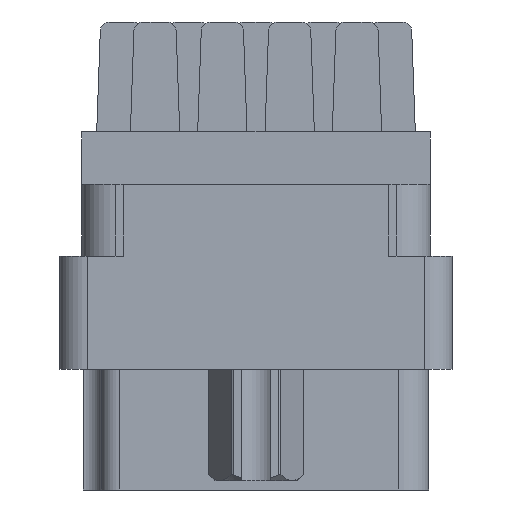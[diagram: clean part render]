
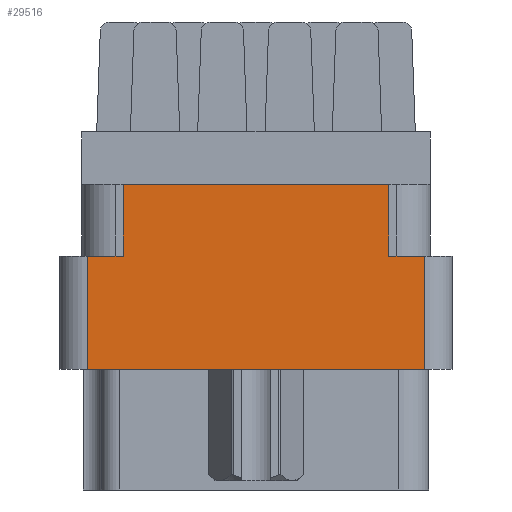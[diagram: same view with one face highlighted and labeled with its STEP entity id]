
A CAD part, left-side view. The second image highlights one B-rep face of the part: STEP entity #29516.
In plain terms, the highlighted planar face has unit normal (-1, 0, 0).
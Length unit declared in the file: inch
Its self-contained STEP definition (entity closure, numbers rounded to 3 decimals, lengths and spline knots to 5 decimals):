
#1002 = LINE ( 'NONE', #26034, #19584 ) ;
#2303 = CARTESIAN_POINT ( 'NONE',  ( -1., 0.376, -0.529 ) ) ;
#3102 = VECTOR ( 'NONE', #3539, 39.37008 ) ;
#3539 = DIRECTION ( 'NONE',  ( 0., -1., 0. ) ) ;
#3864 = CARTESIAN_POINT ( 'NONE',  ( -1., -0.376, -0.277 ) ) ;
#3985 = VECTOR ( 'NONE', #44143, 39.37008 ) ;
#4215 = CARTESIAN_POINT ( 'NONE',  ( -1., -0.438, -0.798 ) ) ;
#5574 = CARTESIAN_POINT ( 'NONE',  ( -1., -0.376, -0.529 ) ) ;
#5891 = VERTEX_POINT ( 'NONE', #5574 ) ;
#5908 = EDGE_CURVE ( 'NONE', #46362, #29553, #9421, .T. ) ;
#5971 = EDGE_CURVE ( 'NONE', #5891, #8321, #36577, .T. ) ;
#6487 = DIRECTION ( 'NONE',  ( 0., 0., -1. ) ) ;
#8308 = FACE_OUTER_BOUND ( 'NONE', #11083, .T. ) ;
#8321 = VERTEX_POINT ( 'NONE', #3864 ) ;
#9182 = CARTESIAN_POINT ( 'NONE',  ( -1., 0., -0.277 ) ) ;
#9421 = LINE ( 'NONE', #9182, #23966 ) ;
#9979 = ORIENTED_EDGE ( 'NONE', *, *, #21699, .F. ) ;
#11083 = EDGE_LOOP ( 'NONE', ( #22367, #42477, #26662, #16470, #28057, #23866, #9979, #14936 ) ) ;
#11517 = EDGE_CURVE ( 'NONE', #46362, #23050, #45489, .T. ) ;
#11698 = CARTESIAN_POINT ( 'NONE',  ( -1., 0.296, -0.277 ) ) ;
#13220 = VECTOR ( 'NONE', #36342, 39.37008 ) ;
#14936 = ORIENTED_EDGE ( 'NONE', *, *, #29615, .F. ) ;
#16118 = LINE ( 'NONE', #30805, #31322 ) ;
#16470 = ORIENTED_EDGE ( 'NONE', *, *, #5971, .T. ) ;
#17505 = VECTOR ( 'NONE', #30531, 39.37008 ) ;
#18346 = CARTESIAN_POINT ( 'NONE',  ( -1., 0.296, -0.117 ) ) ;
#19584 = VECTOR ( 'NONE', #40975, 39.37008 ) ;
#20102 = AXIS2_PLACEMENT_3D ( 'NONE', #4215, #29710, #25619 ) ;
#21337 = VERTEX_POINT ( 'NONE', #22362 ) ;
#21591 = LINE ( 'NONE', #40129, #3102 ) ;
#21699 = EDGE_CURVE ( 'NONE', #25358, #21337, #21591, .T. ) ;
#22362 = CARTESIAN_POINT ( 'NONE',  ( -1., -0.296, -0.117 ) ) ;
#22367 = ORIENTED_EDGE ( 'NONE', *, *, #5908, .F. ) ;
#22500 = LINE ( 'NONE', #33804, #3985 ) ;
#22633 = VERTEX_POINT ( 'NONE', #35212 ) ;
#23050 = VERTEX_POINT ( 'NONE', #2303 ) ;
#23692 = CARTESIAN_POINT ( 'NONE',  ( -1., 0.376, -0.277 ) ) ;
#23845 = DIRECTION ( 'NONE',  ( 0., -1., 0. ) ) ;
#23866 = ORIENTED_EDGE ( 'NONE', *, *, #45884, .T. ) ;
#23966 = VECTOR ( 'NONE', #23845, 39.37008 ) ;
#24549 = CARTESIAN_POINT ( 'NONE',  ( -1., -0.376, -0.798 ) ) ;
#25358 = VERTEX_POINT ( 'NONE', #18346 ) ;
#25619 = DIRECTION ( 'NONE',  ( 0., 0., 1. ) ) ;
#26034 = CARTESIAN_POINT ( 'NONE',  ( -1., 0., -0.529 ) ) ;
#26662 = ORIENTED_EDGE ( 'NONE', *, *, #40275, .F. ) ;
#28057 = ORIENTED_EDGE ( 'NONE', *, *, #39036, .F. ) ;
#29516 = ADVANCED_FACE ( 'NONE', ( #8308 ), #43918, .T. ) ;
#29553 = VERTEX_POINT ( 'NONE', #11698 ) ;
#29615 = EDGE_CURVE ( 'NONE', #29553, #25358, #22500, .T. ) ;
#29710 = DIRECTION ( 'NONE',  ( -1., 0., 0. ) ) ;
#30531 = DIRECTION ( 'NONE',  ( 0., -1., 0. ) ) ;
#30805 = CARTESIAN_POINT ( 'NONE',  ( -1., -0.296, -0.277 ) ) ;
#31031 = DIRECTION ( 'NONE',  ( 0., 0., 1. ) ) ;
#31322 = VECTOR ( 'NONE', #31031, 39.37008 ) ;
#32478 = CARTESIAN_POINT ( 'NONE',  ( -1., 0.376, -0.798 ) ) ;
#33804 = CARTESIAN_POINT ( 'NONE',  ( -1., 0.296, -0.277 ) ) ;
#34137 = LINE ( 'NONE', #45441, #17505 ) ;
#35212 = CARTESIAN_POINT ( 'NONE',  ( -1., -0.296, -0.277 ) ) ;
#36342 = DIRECTION ( 'NONE',  ( 0., 0., 1. ) ) ;
#36577 = LINE ( 'NONE', #24549, #13220 ) ;
#39036 = EDGE_CURVE ( 'NONE', #22633, #8321, #34137, .T. ) ;
#40129 = CARTESIAN_POINT ( 'NONE',  ( -1., 0.438, -0.117 ) ) ;
#40275 = EDGE_CURVE ( 'NONE', #5891, #23050, #1002, .T. ) ;
#40975 = DIRECTION ( 'NONE',  ( 0., 1., 0. ) ) ;
#42477 = ORIENTED_EDGE ( 'NONE', *, *, #11517, .T. ) ;
#43655 = VECTOR ( 'NONE', #6487, 39.37008 ) ;
#43918 = PLANE ( 'NONE',  #20102 ) ;
#44143 = DIRECTION ( 'NONE',  ( 0., 0., 1. ) ) ;
#45441 = CARTESIAN_POINT ( 'NONE',  ( -1., 0., -0.277 ) ) ;
#45489 = LINE ( 'NONE', #32478, #43655 ) ;
#45884 = EDGE_CURVE ( 'NONE', #22633, #21337, #16118, .T. ) ;
#46362 = VERTEX_POINT ( 'NONE', #23692 ) ;
